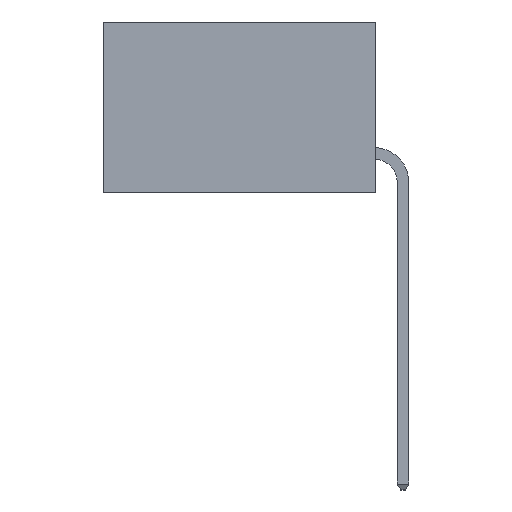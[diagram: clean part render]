
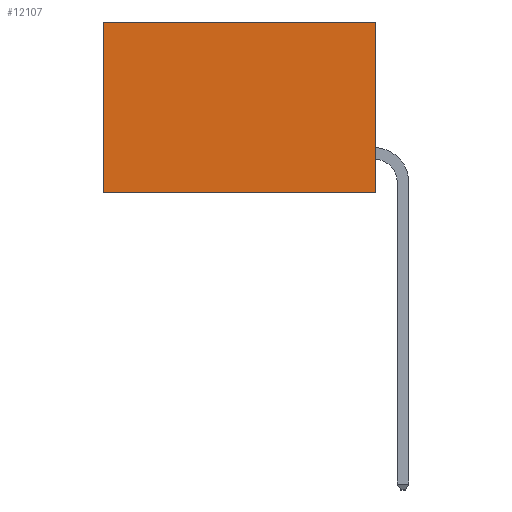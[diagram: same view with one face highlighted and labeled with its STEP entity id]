
A CAD part, left-side view. The second image highlights one B-rep face of the part: STEP entity #12107.
In plain terms, the highlighted planar face has unit normal (-1, 0, 0).
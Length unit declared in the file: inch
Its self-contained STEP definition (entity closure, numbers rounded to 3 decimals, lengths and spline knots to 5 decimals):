
#77 = VERTEX_POINT ( 'NONE', #5570 ) ;
#638 = VECTOR ( 'NONE', #6040, 39.37008 ) ;
#1263 = VERTEX_POINT ( 'NONE', #10019 ) ;
#1408 = ORIENTED_EDGE ( 'NONE', *, *, #4354, .T. ) ;
#2169 = CARTESIAN_POINT ( 'NONE',  ( 0.277, 0., 0. ) ) ;
#2263 = CARTESIAN_POINT ( 'NONE',  ( 0.277, 0., -0.37 ) ) ;
#2580 = ORIENTED_EDGE ( 'NONE', *, *, #6865, .T. ) ;
#2902 = DIRECTION ( 'NONE',  ( 0., 0., -1. ) ) ;
#3535 = LINE ( 'NONE', #2169, #9168 ) ;
#3955 = AXIS2_PLACEMENT_3D ( 'NONE', #2263, #5954, #13823 ) ;
#4354 = EDGE_CURVE ( 'NONE', #6223, #4488, #4864, .T. ) ;
#4391 = CARTESIAN_POINT ( 'NONE',  ( 0.277, 0.59, 0. ) ) ;
#4488 = VERTEX_POINT ( 'NONE', #8057 ) ;
#4864 = LINE ( 'NONE', #11743, #13491 ) ;
#4927 = ORIENTED_EDGE ( 'NONE', *, *, #6176, .F. ) ;
#5116 = DIRECTION ( 'NONE',  ( 0., 0., -1. ) ) ;
#5570 = CARTESIAN_POINT ( 'NONE',  ( 0.277, 0., 0. ) ) ;
#5954 = DIRECTION ( 'NONE',  ( 1., 0., 0. ) ) ;
#6040 = DIRECTION ( 'NONE',  ( 0., 1., 0. ) ) ;
#6077 = CARTESIAN_POINT ( 'NONE',  ( 0.277, 0., -0.37 ) ) ;
#6176 = EDGE_CURVE ( 'NONE', #1263, #4488, #6831, .T. ) ;
#6223 = VERTEX_POINT ( 'NONE', #4391 ) ;
#6831 = LINE ( 'NONE', #6077, #638 ) ;
#6865 = EDGE_CURVE ( 'NONE', #77, #6223, #3535, .T. ) ;
#7903 = ORIENTED_EDGE ( 'NONE', *, *, #9765, .F. ) ;
#8057 = CARTESIAN_POINT ( 'NONE',  ( 0.277, 0.59, -0.37 ) ) ;
#9168 = VECTOR ( 'NONE', #14629, 39.37008 ) ;
#9765 = EDGE_CURVE ( 'NONE', #77, #1263, #11207, .T. ) ;
#10019 = CARTESIAN_POINT ( 'NONE',  ( 0.277, 0., -0.37 ) ) ;
#10820 = CARTESIAN_POINT ( 'NONE',  ( 0.277, 0., -0.37 ) ) ;
#10841 = VECTOR ( 'NONE', #2902, 39.37008 ) ;
#10927 = EDGE_LOOP ( 'NONE', ( #1408, #4927, #7903, #2580 ) ) ;
#11207 = LINE ( 'NONE', #10820, #10841 ) ;
#11743 = CARTESIAN_POINT ( 'NONE',  ( 0.277, 0.59, -0.37 ) ) ;
#12107 = ADVANCED_FACE ( 'NONE', ( #13051 ), #12741, .F. ) ;
#12741 = PLANE ( 'NONE',  #3955 ) ;
#13051 = FACE_OUTER_BOUND ( 'NONE', #10927, .T. ) ;
#13491 = VECTOR ( 'NONE', #5116, 39.37008 ) ;
#13823 = DIRECTION ( 'NONE',  ( 0., 0., -1. ) ) ;
#14629 = DIRECTION ( 'NONE',  ( 0., 1., 0. ) ) ;
